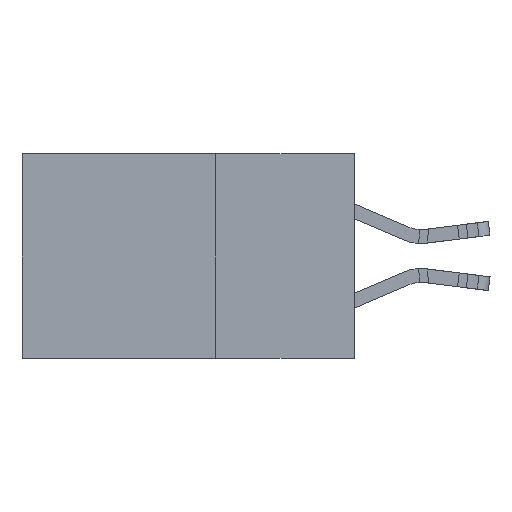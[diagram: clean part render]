
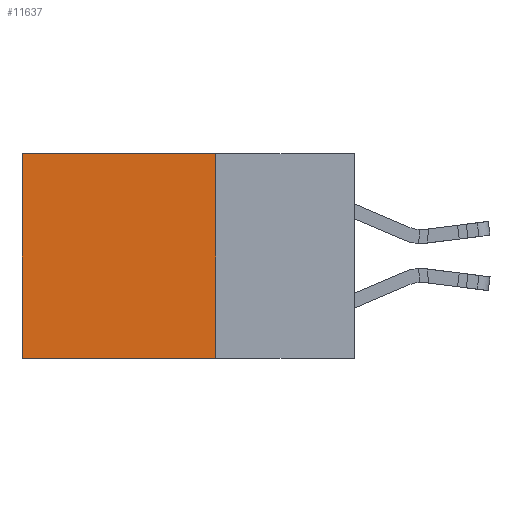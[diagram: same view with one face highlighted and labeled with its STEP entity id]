
A CAD part, left-side view. The second image highlights one B-rep face of the part: STEP entity #11637.
In plain terms, the highlighted planar face has unit normal (-1, 0, 0).
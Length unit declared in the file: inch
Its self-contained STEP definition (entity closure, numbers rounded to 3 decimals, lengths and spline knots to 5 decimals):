
#127 = CARTESIAN_POINT ( 'NONE',  ( 0.2615, 0.6, -0.37 ) ) ;
#656 = CARTESIAN_POINT ( 'NONE',  ( 0.2615, 0.25, -0.37 ) ) ;
#769 = DIRECTION ( 'NONE',  ( 0., 0., -1. ) ) ;
#783 = LINE ( 'NONE', #2598, #10626 ) ;
#1773 = VECTOR ( 'NONE', #20179, 39.37008 ) ;
#2598 = CARTESIAN_POINT ( 'NONE',  ( 0.2615, 0.6, -0.37 ) ) ;
#2641 = VERTEX_POINT ( 'NONE', #127 ) ;
#2737 = VERTEX_POINT ( 'NONE', #14118 ) ;
#3141 = VECTOR ( 'NONE', #3498, 39.37008 ) ;
#3498 = DIRECTION ( 'NONE',  ( 0., 1., 0. ) ) ;
#3595 = FACE_OUTER_BOUND ( 'NONE', #18862, .T. ) ;
#4295 = PLANE ( 'NONE',  #22343 ) ;
#4983 = EDGE_CURVE ( 'NONE', #2737, #8090, #8609, .T. ) ;
#6978 = VERTEX_POINT ( 'NONE', #10021 ) ;
#8007 = DIRECTION ( 'NONE',  ( 0., 0., -1. ) ) ;
#8090 = VERTEX_POINT ( 'NONE', #13731 ) ;
#8609 = LINE ( 'NONE', #15471, #3141 ) ;
#8832 = ORIENTED_EDGE ( 'NONE', *, *, #14161, .F. ) ;
#10021 = CARTESIAN_POINT ( 'NONE',  ( 0.2615, 0.25, -0.37 ) ) ;
#10626 = VECTOR ( 'NONE', #769, 39.37008 ) ;
#11637 = ADVANCED_FACE ( 'NONE', ( #3595 ), #4295, .F. ) ;
#11728 = DIRECTION ( 'NONE',  ( 0., 1., 0. ) ) ;
#12413 = EDGE_CURVE ( 'NONE', #6978, #2641, #22820, .T. ) ;
#13125 = VECTOR ( 'NONE', #11728, 39.37008 ) ;
#13731 = CARTESIAN_POINT ( 'NONE',  ( 0.2615, 0.6, 0. ) ) ;
#14118 = CARTESIAN_POINT ( 'NONE',  ( 0.2615, 0.25, 0. ) ) ;
#14161 = EDGE_CURVE ( 'NONE', #2737, #6978, #16478, .T. ) ;
#14215 = ORIENTED_EDGE ( 'NONE', *, *, #16359, .T. ) ;
#15471 = CARTESIAN_POINT ( 'NONE',  ( 0.2615, 0.25, 0. ) ) ;
#16359 = EDGE_CURVE ( 'NONE', #8090, #2641, #783, .T. ) ;
#16478 = LINE ( 'NONE', #16491, #1773 ) ;
#16491 = CARTESIAN_POINT ( 'NONE',  ( 0.2615, 0.25, -0.37 ) ) ;
#17154 = CARTESIAN_POINT ( 'NONE',  ( 0.2615, 0.25, -0.37 ) ) ;
#18862 = EDGE_LOOP ( 'NONE', ( #14215, #22498, #8832, #19461 ) ) ;
#19025 = DIRECTION ( 'NONE',  ( 1., 0., 0. ) ) ;
#19461 = ORIENTED_EDGE ( 'NONE', *, *, #4983, .T. ) ;
#20179 = DIRECTION ( 'NONE',  ( 0., 0., -1. ) ) ;
#22343 = AXIS2_PLACEMENT_3D ( 'NONE', #17154, #19025, #8007 ) ;
#22498 = ORIENTED_EDGE ( 'NONE', *, *, #12413, .F. ) ;
#22820 = LINE ( 'NONE', #656, #13125 ) ;
